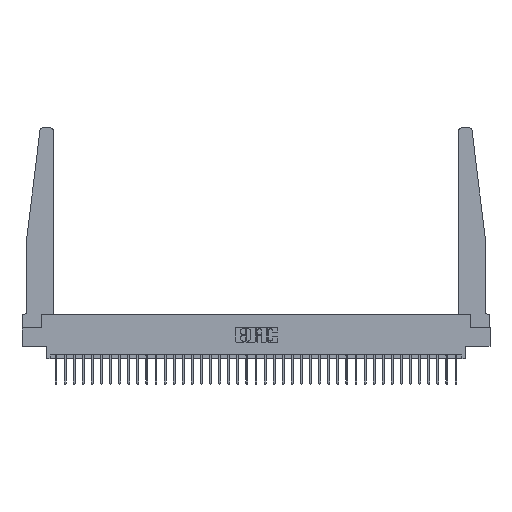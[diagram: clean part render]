
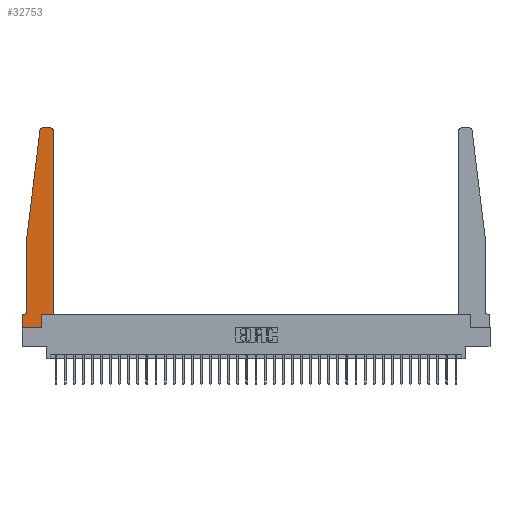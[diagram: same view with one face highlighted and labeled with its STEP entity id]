
A CAD part, top view. The second image highlights one B-rep face of the part: STEP entity #32753.
In plain terms, the highlighted planar face has unit normal (0, 0, 1).
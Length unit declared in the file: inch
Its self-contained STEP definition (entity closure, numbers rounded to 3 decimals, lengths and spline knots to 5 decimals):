
#594 = EDGE_CURVE ( 'NONE', #7757, #11420, #3836, .T. ) ;
#668 = VERTEX_POINT ( 'NONE', #5612 ) ;
#1547 = LINE ( 'NONE', #22759, #13828 ) ;
#2252 = ORIENTED_EDGE ( 'NONE', *, *, #14410, .T. ) ;
#2482 = VERTEX_POINT ( 'NONE', #10802 ) ;
#2628 = VERTEX_POINT ( 'NONE', #24395 ) ;
#2712 = AXIS2_PLACEMENT_3D ( 'NONE', #28584, #12877, #31193 ) ;
#2928 = CARTESIAN_POINT ( 'NONE',  ( 0., 0., 0.37 ) ) ;
#3053 = CARTESIAN_POINT ( 'NONE',  ( 0.24675, 2.72367, 0.37 ) ) ;
#3110 = EDGE_CURVE ( 'NONE', #23674, #16459, #33579, .T. ) ;
#3159 = ORIENTED_EDGE ( 'NONE', *, *, #33346, .T. ) ;
#3385 = CARTESIAN_POINT ( 'NONE',  ( 0.065, 0.1875, 0.37 ) ) ;
#3836 = LINE ( 'NONE', #5276, #30877 ) ;
#4508 = CARTESIAN_POINT ( 'NONE',  ( 0.2605, 0., 0.37 ) ) ;
#4536 = CARTESIAN_POINT ( 'NONE',  ( 0.015, 0.2375, 0.37 ) ) ;
#4612 = EDGE_CURVE ( 'NONE', #24198, #2482, #27685, .T. ) ;
#5276 = CARTESIAN_POINT ( 'NONE',  ( 0.065, 1.25, 0.37 ) ) ;
#5612 = CARTESIAN_POINT ( 'NONE',  ( 0.425, 0.18, 0.37 ) ) ;
#5675 = CARTESIAN_POINT ( 'NONE',  ( 0.065, 0.2375, 0.37 ) ) ;
#5747 = DIRECTION ( 'NONE',  ( 0., 0., 1. ) ) ;
#6220 = LINE ( 'NONE', #26987, #26339 ) ;
#6277 = ORIENTED_EDGE ( 'NONE', *, *, #25443, .T. ) ;
#6752 = VECTOR ( 'NONE', #16457, 39.37008 ) ;
#6860 = CARTESIAN_POINT ( 'NONE',  ( 0., 0.1875, 0.37 ) ) ;
#7165 = DIRECTION ( 'NONE',  ( -1., 0., 0. ) ) ;
#7326 = VECTOR ( 'NONE', #30225, 39.37008 ) ;
#7680 = VECTOR ( 'NONE', #26610, 39.37008 ) ;
#7757 = VERTEX_POINT ( 'NONE', #3053 ) ;
#7806 = CARTESIAN_POINT ( 'NONE',  ( 0.065, 1.25, 0.37 ) ) ;
#8154 = LINE ( 'NONE', #32866, #7326 ) ;
#8339 = CARTESIAN_POINT ( 'NONE',  ( 0.25, 2.75, 0.37 ) ) ;
#8622 = AXIS2_PLACEMENT_3D ( 'NONE', #4536, #22857, #7165 ) ;
#9314 = VERTEX_POINT ( 'NONE', #27363 ) ;
#10381 = EDGE_CURVE ( 'NONE', #668, #9314, #27761, .T. ) ;
#10802 = CARTESIAN_POINT ( 'NONE',  ( 0.27653, 2.75, 0.37 ) ) ;
#10889 = CARTESIAN_POINT ( 'NONE',  ( 0., 0., 0.37 ) ) ;
#11056 = ORIENTED_EDGE ( 'NONE', *, *, #594, .T. ) ;
#11420 = VERTEX_POINT ( 'NONE', #7806 ) ;
#11640 = EDGE_CURVE ( 'NONE', #22150, #2628, #6220, .T. ) ;
#11669 = LINE ( 'NONE', #33388, #17812 ) ;
#11826 = FACE_OUTER_BOUND ( 'NONE', #23074, .T. ) ;
#12434 = DIRECTION ( 'NONE',  ( 0., -1., 0. ) ) ;
#12663 = AXIS2_PLACEMENT_3D ( 'NONE', #21445, #5747, #24075 ) ;
#12672 = ORIENTED_EDGE ( 'NONE', *, *, #3110, .T. ) ;
#12809 = CARTESIAN_POINT ( 'NONE',  ( 0.395, 2.75, 0.37 ) ) ;
#12877 = DIRECTION ( 'NONE',  ( 0., 0., 1. ) ) ;
#13480 = AXIS2_PLACEMENT_3D ( 'NONE', #6860, #33089, #17408 ) ;
#13828 = VECTOR ( 'NONE', #25418, 39.37008 ) ;
#14410 = EDGE_CURVE ( 'NONE', #26687, #22150, #8154, .T. ) ;
#14534 = LINE ( 'NONE', #3385, #6752 ) ;
#14545 = VECTOR ( 'NONE', #26688, 39.37008 ) ;
#14984 = EDGE_CURVE ( 'NONE', #9314, #24198, #31861, .T. ) ;
#15204 = LINE ( 'NONE', #2928, #28331 ) ;
#15821 = DIRECTION ( 'NONE',  ( -0.122, -0.992, 0. ) ) ;
#16130 = CARTESIAN_POINT ( 'NONE',  ( 0.015, 0.1875, 0.37 ) ) ;
#16457 = DIRECTION ( 'NONE',  ( -1., 0., 0. ) ) ;
#16459 = VERTEX_POINT ( 'NONE', #16130 ) ;
#16908 = EDGE_CURVE ( 'NONE', #11420, #23674, #11669, .T. ) ;
#17408 = DIRECTION ( 'NONE',  ( 1., 0., 0. ) ) ;
#17812 = VECTOR ( 'NONE', #12434, 39.37008 ) ;
#18183 = EDGE_CURVE ( 'NONE', #16459, #29695, #14534, .T. ) ;
#18680 = CARTESIAN_POINT ( 'NONE',  ( 0.425, 0.18, 0.37 ) ) ;
#19359 = ORIENTED_EDGE ( 'NONE', *, *, #31211, .T. ) ;
#21445 = CARTESIAN_POINT ( 'NONE',  ( 0.27653, 2.72, 0.37 ) ) ;
#22150 = VERTEX_POINT ( 'NONE', #4508 ) ;
#22759 = CARTESIAN_POINT ( 'NONE',  ( 0.425, 0.18, 0.37 ) ) ;
#22857 = DIRECTION ( 'NONE',  ( 0., 0., -1. ) ) ;
#23074 = EDGE_LOOP ( 'NONE', ( #26722, #6277, #11056, #23362, #12672, #25520, #19359, #2252, #27386, #3159, #28567, #28226 ) ) ;
#23362 = ORIENTED_EDGE ( 'NONE', *, *, #16908, .T. ) ;
#23674 = VERTEX_POINT ( 'NONE', #5675 ) ;
#24075 = DIRECTION ( 'NONE',  ( 1., 0., 0. ) ) ;
#24136 = CARTESIAN_POINT ( 'NONE',  ( 0., 0.1875, 0.37 ) ) ;
#24198 = VERTEX_POINT ( 'NONE', #12809 ) ;
#24395 = CARTESIAN_POINT ( 'NONE',  ( 0.2605, 0.18, 0.37 ) ) ;
#25418 = DIRECTION ( 'NONE',  ( 1., 0., 0. ) ) ;
#25443 = EDGE_CURVE ( 'NONE', #2482, #7757, #30556, .T. ) ;
#25520 = ORIENTED_EDGE ( 'NONE', *, *, #18183, .T. ) ;
#26339 = VECTOR ( 'NONE', #29613, 39.37008 ) ;
#26610 = DIRECTION ( 'NONE',  ( 0., 1., 0. ) ) ;
#26687 = VERTEX_POINT ( 'NONE', #10889 ) ;
#26688 = DIRECTION ( 'NONE',  ( -1., 0., 0. ) ) ;
#26722 = ORIENTED_EDGE ( 'NONE', *, *, #4612, .T. ) ;
#26987 = CARTESIAN_POINT ( 'NONE',  ( 0.2605, 0.18, 0.37 ) ) ;
#27363 = CARTESIAN_POINT ( 'NONE',  ( 0.425, 2.72, 0.37 ) ) ;
#27386 = ORIENTED_EDGE ( 'NONE', *, *, #11640, .T. ) ;
#27685 = LINE ( 'NONE', #8339, #14545 ) ;
#27761 = LINE ( 'NONE', #18680, #7680 ) ;
#28226 = ORIENTED_EDGE ( 'NONE', *, *, #14984, .T. ) ;
#28331 = VECTOR ( 'NONE', #29153, 39.37008 ) ;
#28567 = ORIENTED_EDGE ( 'NONE', *, *, #10381, .T. ) ;
#28584 = CARTESIAN_POINT ( 'NONE',  ( 0.395, 2.72, 0.37 ) ) ;
#29153 = DIRECTION ( 'NONE',  ( 0., -1., 0. ) ) ;
#29613 = DIRECTION ( 'NONE',  ( 0., 1., 0. ) ) ;
#29695 = VERTEX_POINT ( 'NONE', #24136 ) ;
#30225 = DIRECTION ( 'NONE',  ( 1., 0., 0. ) ) ;
#30451 = PLANE ( 'NONE',  #13480 ) ;
#30556 = CIRCLE ( 'NONE', #12663, 0.03 ) ;
#30877 = VECTOR ( 'NONE', #15821, 39.37008 ) ;
#31193 = DIRECTION ( 'NONE',  ( 1., 0., 0. ) ) ;
#31211 = EDGE_CURVE ( 'NONE', #29695, #26687, #15204, .T. ) ;
#31861 = CIRCLE ( 'NONE', #2712, 0.03 ) ;
#32753 = ADVANCED_FACE ( 'NONE', ( #11826 ), #30451, .T. ) ;
#32866 = CARTESIAN_POINT ( 'NONE',  ( 0., 0., 0.37 ) ) ;
#33089 = DIRECTION ( 'NONE',  ( 0., 0., 1. ) ) ;
#33346 = EDGE_CURVE ( 'NONE', #2628, #668, #1547, .T. ) ;
#33388 = CARTESIAN_POINT ( 'NONE',  ( 0.065, 1.25, 0.37 ) ) ;
#33579 = CIRCLE ( 'NONE', #8622, 0.05 ) ;
